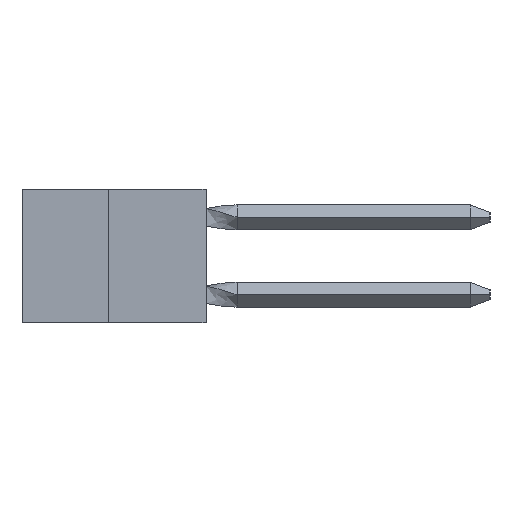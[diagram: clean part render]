
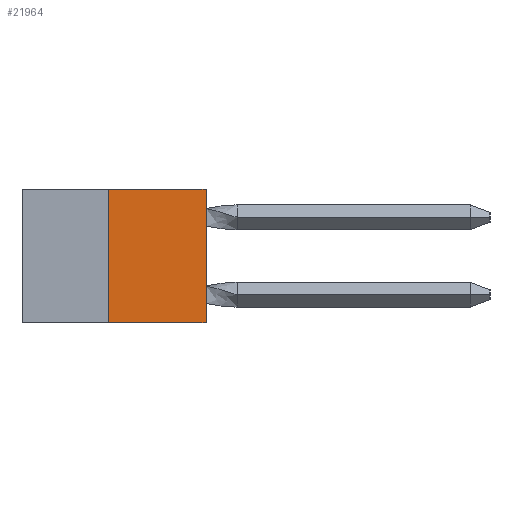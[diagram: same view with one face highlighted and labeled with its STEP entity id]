
A CAD part, left-side view. The second image highlights one B-rep face of the part: STEP entity #21964.
In plain terms, the highlighted planar face has unit normal (-1, 0, 0).
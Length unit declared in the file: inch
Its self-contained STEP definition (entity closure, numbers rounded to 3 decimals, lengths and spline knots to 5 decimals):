
#200 = LINE ( 'NONE', #34842, #35835 ) ;
#1379 = VERTEX_POINT ( 'NONE', #9149 ) ;
#3309 = CARTESIAN_POINT ( 'NONE',  ( 0., 0., -0.343 ) ) ;
#3395 = EDGE_CURVE ( 'NONE', #31168, #10045, #6739, .T. ) ;
#4905 = FACE_OUTER_BOUND ( 'NONE', #6882, .T. ) ;
#6739 = LINE ( 'NONE', #23756, #11735 ) ;
#6882 = EDGE_LOOP ( 'NONE', ( #43239, #29035, #14501, #33128 ) ) ;
#7176 = EDGE_CURVE ( 'NONE', #33867, #31168, #11156, .T. ) ;
#9149 = CARTESIAN_POINT ( 'NONE',  ( 0., 0.25, 0. ) ) ;
#10045 = VERTEX_POINT ( 'NONE', #22164 ) ;
#10576 = DIRECTION ( 'NONE',  ( 0., -1., 0. ) ) ;
#11156 = LINE ( 'NONE', #21524, #36274 ) ;
#11735 = VECTOR ( 'NONE', #16081, 39.37008 ) ;
#14253 = VECTOR ( 'NONE', #33057, 39.37008 ) ;
#14501 = ORIENTED_EDGE ( 'NONE', *, *, #7176, .T. ) ;
#16081 = DIRECTION ( 'NONE',  ( 0., 0., 1. ) ) ;
#16275 = DIRECTION ( 'NONE',  ( 1., 0., 0. ) ) ;
#17062 = CARTESIAN_POINT ( 'NONE',  ( 0., 0.25, -0.343 ) ) ;
#21524 = CARTESIAN_POINT ( 'NONE',  ( 0., 0.473, -0.343 ) ) ;
#21964 = ADVANCED_FACE ( 'NONE', ( #4905 ), #44632, .F. ) ;
#22164 = CARTESIAN_POINT ( 'NONE',  ( 0., 0., 0. ) ) ;
#22282 = CARTESIAN_POINT ( 'NONE',  ( 0., 0.473, 0. ) ) ;
#23756 = CARTESIAN_POINT ( 'NONE',  ( 0., 0., 0. ) ) ;
#26724 = DIRECTION ( 'NONE',  ( 0., 0., -1. ) ) ;
#29035 = ORIENTED_EDGE ( 'NONE', *, *, #43393, .F. ) ;
#30258 = AXIS2_PLACEMENT_3D ( 'NONE', #44479, #16275, #26724 ) ;
#31168 = VERTEX_POINT ( 'NONE', #3309 ) ;
#33057 = DIRECTION ( 'NONE',  ( 0., -1., 0. ) ) ;
#33128 = ORIENTED_EDGE ( 'NONE', *, *, #3395, .T. ) ;
#33867 = VERTEX_POINT ( 'NONE', #17062 ) ;
#34842 = CARTESIAN_POINT ( 'NONE',  ( 0., 0.25, 0. ) ) ;
#35835 = VECTOR ( 'NONE', #38582, 39.37008 ) ;
#36274 = VECTOR ( 'NONE', #10576, 39.37008 ) ;
#38582 = DIRECTION ( 'NONE',  ( 0., 0., 1. ) ) ;
#40941 = EDGE_CURVE ( 'NONE', #1379, #10045, #45461, .T. ) ;
#43239 = ORIENTED_EDGE ( 'NONE', *, *, #40941, .F. ) ;
#43393 = EDGE_CURVE ( 'NONE', #33867, #1379, #200, .T. ) ;
#44479 = CARTESIAN_POINT ( 'NONE',  ( 0., 0.473, 0. ) ) ;
#44632 = PLANE ( 'NONE',  #30258 ) ;
#45461 = LINE ( 'NONE', #22282, #14253 ) ;
